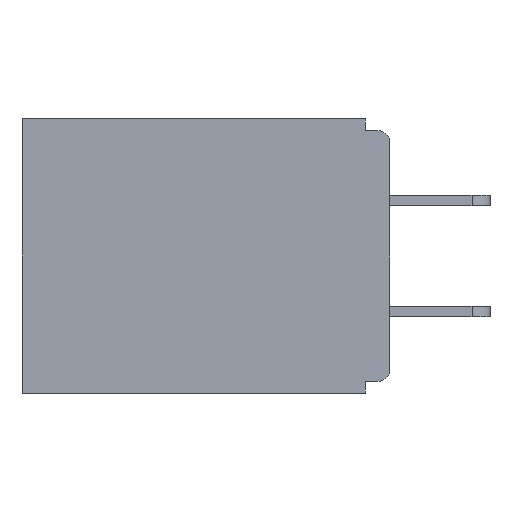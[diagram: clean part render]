
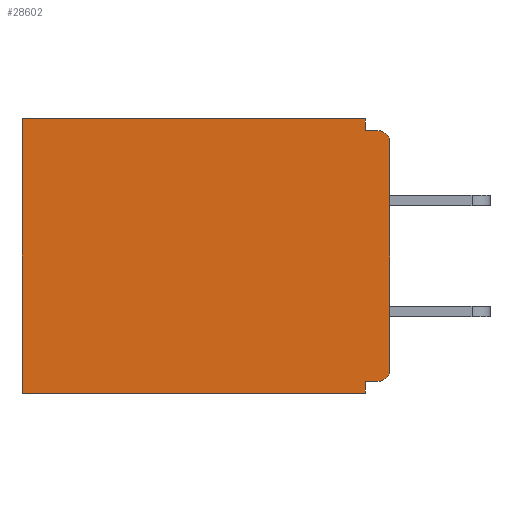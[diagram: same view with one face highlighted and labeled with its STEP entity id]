
A CAD part, left-side view. The second image highlights one B-rep face of the part: STEP entity #28602.
In plain terms, the highlighted planar face has unit normal (-1, 0, 0).
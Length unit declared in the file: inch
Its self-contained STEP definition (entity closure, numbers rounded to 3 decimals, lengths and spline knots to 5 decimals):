
#145 = PLANE ( 'NONE',  #25551 ) ;
#290 = LINE ( 'NONE', #12101, #11044 ) ;
#413 = CARTESIAN_POINT ( 'NONE',  ( 0.298, 0.015, -0.03 ) ) ;
#956 = CIRCLE ( 'NONE', #27770, 0.015 ) ;
#1796 = DIRECTION ( 'NONE',  ( 0., 0., -1. ) ) ;
#1839 = VECTOR ( 'NONE', #14525, 39.37008 ) ;
#2355 = VERTEX_POINT ( 'NONE', #3107 ) ;
#2476 = DIRECTION ( 'NONE',  ( 0., 0., -1. ) ) ;
#2575 = EDGE_CURVE ( 'NONE', #16564, #9519, #15762, .T. ) ;
#3069 = EDGE_CURVE ( 'NONE', #26805, #26217, #3694, .T. ) ;
#3070 = DIRECTION ( 'NONE',  ( 0., -1., 0. ) ) ;
#3107 = CARTESIAN_POINT ( 'NONE',  ( 0.298, 0.031, -0.015 ) ) ;
#3694 = CIRCLE ( 'NONE', #19916, 0.015 ) ;
#4333 = CARTESIAN_POINT ( 'NONE',  ( 0.298, 0.031, -0.328 ) ) ;
#4560 = LINE ( 'NONE', #16271, #26038 ) ;
#5018 = ORIENTED_EDGE ( 'NONE', *, *, #15895, .F. ) ;
#5135 = CARTESIAN_POINT ( 'NONE',  ( 0.298, 0.46, -0.343 ) ) ;
#5386 = VERTEX_POINT ( 'NONE', #17280 ) ;
#5465 = VECTOR ( 'NONE', #9001, 39.37008 ) ;
#5836 = EDGE_CURVE ( 'NONE', #2355, #11504, #4560, .T. ) ;
#6231 = FACE_OUTER_BOUND ( 'NONE', #9458, .T. ) ;
#6604 = CARTESIAN_POINT ( 'NONE',  ( 0.298, 0., -0.328 ) ) ;
#6718 = VERTEX_POINT ( 'NONE', #14854 ) ;
#6956 = DIRECTION ( 'NONE',  ( 1., 0., 0. ) ) ;
#7300 = DIRECTION ( 'NONE',  ( 0., 1., 0. ) ) ;
#8028 = VECTOR ( 'NONE', #17902, 39.37008 ) ;
#8965 = DIRECTION ( 'NONE',  ( -1., 0., 0. ) ) ;
#9001 = DIRECTION ( 'NONE',  ( 0., 0., -1. ) ) ;
#9151 = ORIENTED_EDGE ( 'NONE', *, *, #18519, .T. ) ;
#9458 = EDGE_LOOP ( 'NONE', ( #9151, #11074, #16934, #25746, #16112, #5018, #28573, #17539, #22237, #15084 ) ) ;
#9519 = VERTEX_POINT ( 'NONE', #24467 ) ;
#10029 = VECTOR ( 'NONE', #7300, 39.37008 ) ;
#10782 = CARTESIAN_POINT ( 'NONE',  ( 0.298, 0., -0.313 ) ) ;
#10976 = EDGE_CURVE ( 'NONE', #26805, #16564, #13894, .T. ) ;
#11044 = VECTOR ( 'NONE', #19060, 39.37008 ) ;
#11074 = ORIENTED_EDGE ( 'NONE', *, *, #5836, .F. ) ;
#11129 = CARTESIAN_POINT ( 'NONE',  ( 0.298, 0.015, -0.328 ) ) ;
#11310 = CARTESIAN_POINT ( 'NONE',  ( 0.298, 0.015, -0.015 ) ) ;
#11504 = VERTEX_POINT ( 'NONE', #11310 ) ;
#11859 = VECTOR ( 'NONE', #1796, 39.37008 ) ;
#11944 = VERTEX_POINT ( 'NONE', #21220 ) ;
#12101 = CARTESIAN_POINT ( 'NONE',  ( 0.298, 0.031, -0.343 ) ) ;
#12303 = EDGE_CURVE ( 'NONE', #6718, #11944, #12429, .T. ) ;
#12423 = EDGE_CURVE ( 'NONE', #6718, #2355, #290, .T. ) ;
#12429 = LINE ( 'NONE', #18405, #10029 ) ;
#12942 = VERTEX_POINT ( 'NONE', #5135 ) ;
#13894 = LINE ( 'NONE', #6604, #8028 ) ;
#14525 = DIRECTION ( 'NONE',  ( 0., 1., 0. ) ) ;
#14854 = CARTESIAN_POINT ( 'NONE',  ( 0.298, 0.031, 0. ) ) ;
#15032 = CARTESIAN_POINT ( 'NONE',  ( 0.298, 0.46, 0. ) ) ;
#15084 = ORIENTED_EDGE ( 'NONE', *, *, #25118, .F. ) ;
#15149 = CARTESIAN_POINT ( 'NONE',  ( 0.298, 0.031, -0.343 ) ) ;
#15378 = EDGE_CURVE ( 'NONE', #11944, #12942, #21209, .T. ) ;
#15434 = DIRECTION ( 'NONE',  ( 0., 0., -1. ) ) ;
#15762 = LINE ( 'NONE', #15149, #21658 ) ;
#15895 = EDGE_CURVE ( 'NONE', #9519, #12942, #19480, .T. ) ;
#16112 = ORIENTED_EDGE ( 'NONE', *, *, #15378, .T. ) ;
#16271 = CARTESIAN_POINT ( 'NONE',  ( 0.298, 0., -0.015 ) ) ;
#16564 = VERTEX_POINT ( 'NONE', #4333 ) ;
#16934 = ORIENTED_EDGE ( 'NONE', *, *, #12423, .F. ) ;
#17280 = CARTESIAN_POINT ( 'NONE',  ( 0.298, 0., -0.03 ) ) ;
#17539 = ORIENTED_EDGE ( 'NONE', *, *, #10976, .F. ) ;
#17902 = DIRECTION ( 'NONE',  ( 0., 1., 0. ) ) ;
#18405 = CARTESIAN_POINT ( 'NONE',  ( 0.298, 0., 0. ) ) ;
#18519 = EDGE_CURVE ( 'NONE', #5386, #11504, #956, .T. ) ;
#18875 = CARTESIAN_POINT ( 'NONE',  ( 0.298, 0., -0.343 ) ) ;
#19060 = DIRECTION ( 'NONE',  ( 0., 0., -1. ) ) ;
#19480 = LINE ( 'NONE', #18875, #1839 ) ;
#19916 = AXIS2_PLACEMENT_3D ( 'NONE', #20912, #23068, #25702 ) ;
#20912 = CARTESIAN_POINT ( 'NONE',  ( 0.298, 0.015, -0.313 ) ) ;
#21209 = LINE ( 'NONE', #15032, #11859 ) ;
#21220 = CARTESIAN_POINT ( 'NONE',  ( 0.298, 0.46, 0. ) ) ;
#21638 = DIRECTION ( 'NONE',  ( 0., 0., -1. ) ) ;
#21658 = VECTOR ( 'NONE', #21638, 39.37008 ) ;
#22237 = ORIENTED_EDGE ( 'NONE', *, *, #3069, .T. ) ;
#23068 = DIRECTION ( 'NONE',  ( -1., 0., 0. ) ) ;
#24251 = CARTESIAN_POINT ( 'NONE',  ( 0.298, 0., 0. ) ) ;
#24467 = CARTESIAN_POINT ( 'NONE',  ( 0.298, 0.031, -0.343 ) ) ;
#25118 = EDGE_CURVE ( 'NONE', #5386, #26217, #27675, .T. ) ;
#25551 = AXIS2_PLACEMENT_3D ( 'NONE', #24251, #6956, #15434 ) ;
#25702 = DIRECTION ( 'NONE',  ( 0., 0., -1. ) ) ;
#25746 = ORIENTED_EDGE ( 'NONE', *, *, #12303, .T. ) ;
#26038 = VECTOR ( 'NONE', #3070, 39.37008 ) ;
#26217 = VERTEX_POINT ( 'NONE', #10782 ) ;
#26538 = CARTESIAN_POINT ( 'NONE',  ( 0.298, 0., 0. ) ) ;
#26805 = VERTEX_POINT ( 'NONE', #11129 ) ;
#27675 = LINE ( 'NONE', #26538, #5465 ) ;
#27770 = AXIS2_PLACEMENT_3D ( 'NONE', #413, #8965, #2476 ) ;
#28573 = ORIENTED_EDGE ( 'NONE', *, *, #2575, .F. ) ;
#28602 = ADVANCED_FACE ( 'NONE', ( #6231 ), #145, .F. ) ;
